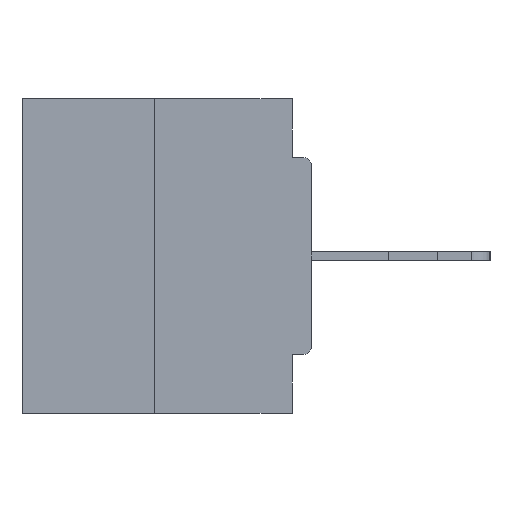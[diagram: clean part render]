
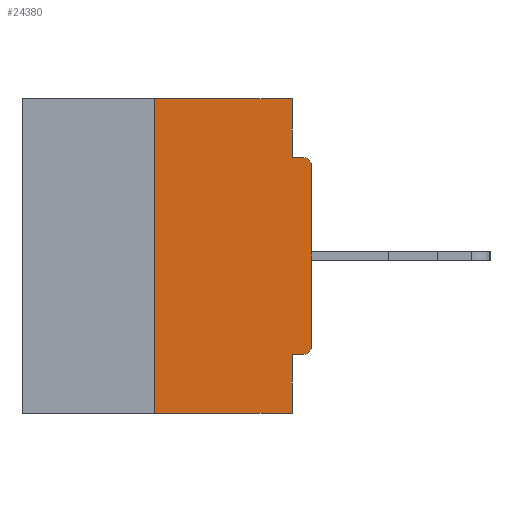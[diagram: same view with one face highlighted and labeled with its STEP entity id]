
A CAD part, left-side view. The second image highlights one B-rep face of the part: STEP entity #24380.
In plain terms, the highlighted planar face has unit normal (-1, 0, 0).
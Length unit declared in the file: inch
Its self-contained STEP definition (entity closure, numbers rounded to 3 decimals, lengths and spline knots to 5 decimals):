
#526 = ORIENTED_EDGE ( 'NONE', *, *, #13476, .T. ) ;
#1643 = DIRECTION ( 'NONE',  ( 0., 0., -1. ) ) ;
#1683 = CARTESIAN_POINT ( 'NONE',  ( 0., 0.46, 0. ) ) ;
#2128 = CARTESIAN_POINT ( 'NONE',  ( 0., 0.015, -0.4065 ) ) ;
#3144 = DIRECTION ( 'NONE',  ( 0., 1., 0. ) ) ;
#4366 = EDGE_CURVE ( 'NONE', #31973, #18933, #22867, .T. ) ;
#4422 = VERTEX_POINT ( 'NONE', #16410 ) ;
#5342 = VECTOR ( 'NONE', #16823, 39.37008 ) ;
#6203 = CARTESIAN_POINT ( 'NONE',  ( 0., 0.46, -0.5 ) ) ;
#6242 = ORIENTED_EDGE ( 'NONE', *, *, #23953, .F. ) ;
#6305 = PLANE ( 'NONE',  #9813 ) ;
#6490 = DIRECTION ( 'NONE',  ( 0., 0., -1. ) ) ;
#6770 = EDGE_LOOP ( 'NONE', ( #6242, #31537, #29741, #21243, #16342, #526, #17858, #17144, #28918, #13079 ) ) ;
#6972 = VECTOR ( 'NONE', #21790, 39.37008 ) ;
#6973 = LINE ( 'NONE', #30131, #22857 ) ;
#7571 = CARTESIAN_POINT ( 'NONE',  ( 0., 0., -0.1085 ) ) ;
#7632 = LINE ( 'NONE', #1683, #5342 ) ;
#8590 = VERTEX_POINT ( 'NONE', #9609 ) ;
#8731 = CARTESIAN_POINT ( 'NONE',  ( 0., 0.031, -0.4065 ) ) ;
#8762 = CARTESIAN_POINT ( 'NONE',  ( 0., 0.46, 0. ) ) ;
#8994 = CARTESIAN_POINT ( 'NONE',  ( 0., 0.015, -0.1085 ) ) ;
#9557 = EDGE_CURVE ( 'NONE', #23569, #20848, #27649, .T. ) ;
#9609 = CARTESIAN_POINT ( 'NONE',  ( 0., 0.031, -0.5 ) ) ;
#9813 = AXIS2_PLACEMENT_3D ( 'NONE', #8762, #31168, #1643 ) ;
#10285 = VERTEX_POINT ( 'NONE', #24629 ) ;
#10954 = CARTESIAN_POINT ( 'NONE',  ( 0., 0.25, 0. ) ) ;
#11067 = LINE ( 'NONE', #27284, #30048 ) ;
#12537 = CARTESIAN_POINT ( 'NONE',  ( 0., 0.031, -0.0935 ) ) ;
#13079 = ORIENTED_EDGE ( 'NONE', *, *, #22885, .F. ) ;
#13197 = VECTOR ( 'NONE', #15834, 39.37008 ) ;
#13476 = EDGE_CURVE ( 'NONE', #31973, #10285, #26076, .T. ) ;
#13555 = LINE ( 'NONE', #17165, #6972 ) ;
#13571 = VECTOR ( 'NONE', #3144, 39.37008 ) ;
#13758 = DIRECTION ( 'NONE',  ( 0., 0., 1. ) ) ;
#13796 = FACE_OUTER_BOUND ( 'NONE', #6770, .T. ) ;
#14166 = CARTESIAN_POINT ( 'NONE',  ( 0., 0.015, -0.3915 ) ) ;
#14942 = EDGE_CURVE ( 'NONE', #22138, #22860, #22891, .T. ) ;
#15296 = AXIS2_PLACEMENT_3D ( 'NONE', #8994, #31083, #6490 ) ;
#15401 = DIRECTION ( 'NONE',  ( 0., 0., -1. ) ) ;
#15822 = VERTEX_POINT ( 'NONE', #7571 ) ;
#15834 = DIRECTION ( 'NONE',  ( 0., -1., 0. ) ) ;
#16342 = ORIENTED_EDGE ( 'NONE', *, *, #4366, .F. ) ;
#16410 = CARTESIAN_POINT ( 'NONE',  ( 0., 0.031, 0. ) ) ;
#16823 = DIRECTION ( 'NONE',  ( 0., -1., 0. ) ) ;
#16846 = CIRCLE ( 'NONE', #15296, 0.015 ) ;
#17144 = ORIENTED_EDGE ( 'NONE', *, *, #28831, .T. ) ;
#17165 = CARTESIAN_POINT ( 'NONE',  ( 0., 0.031, -0.5 ) ) ;
#17858 = ORIENTED_EDGE ( 'NONE', *, *, #22026, .T. ) ;
#18138 = VECTOR ( 'NONE', #21350, 39.37008 ) ;
#18157 = EDGE_CURVE ( 'NONE', #18933, #8590, #13555, .T. ) ;
#18933 = VERTEX_POINT ( 'NONE', #8731 ) ;
#19499 = DIRECTION ( 'NONE',  ( 0., 0., 1. ) ) ;
#20848 = VERTEX_POINT ( 'NONE', #22329 ) ;
#21243 = ORIENTED_EDGE ( 'NONE', *, *, #18157, .F. ) ;
#21350 = DIRECTION ( 'NONE',  ( 0., -1., 0. ) ) ;
#21579 = AXIS2_PLACEMENT_3D ( 'NONE', #14166, #31510, #29457 ) ;
#21790 = DIRECTION ( 'NONE',  ( 0., 0., -1. ) ) ;
#22026 = EDGE_CURVE ( 'NONE', #10285, #15822, #11067, .T. ) ;
#22138 = VERTEX_POINT ( 'NONE', #12537 ) ;
#22329 = CARTESIAN_POINT ( 'NONE',  ( 0., 0.25, 0. ) ) ;
#22857 = VECTOR ( 'NONE', #15401, 39.37008 ) ;
#22860 = VERTEX_POINT ( 'NONE', #22880 ) ;
#22867 = LINE ( 'NONE', #30288, #13571 ) ;
#22880 = CARTESIAN_POINT ( 'NONE',  ( 0., 0.015, -0.0935 ) ) ;
#22885 = EDGE_CURVE ( 'NONE', #4422, #22138, #6973, .T. ) ;
#22891 = LINE ( 'NONE', #30683, #13197 ) ;
#23569 = VERTEX_POINT ( 'NONE', #24794 ) ;
#23771 = EDGE_CURVE ( 'NONE', #23569, #8590, #28168, .T. ) ;
#23953 = EDGE_CURVE ( 'NONE', #20848, #4422, #7632, .T. ) ;
#24380 = ADVANCED_FACE ( 'NONE', ( #13796 ), #6305, .F. ) ;
#24629 = CARTESIAN_POINT ( 'NONE',  ( 0., 0., -0.3915 ) ) ;
#24794 = CARTESIAN_POINT ( 'NONE',  ( 0., 0.25, -0.5 ) ) ;
#26076 = CIRCLE ( 'NONE', #21579, 0.015 ) ;
#27284 = CARTESIAN_POINT ( 'NONE',  ( 0., 0., 0. ) ) ;
#27649 = LINE ( 'NONE', #10954, #31910 ) ;
#28168 = LINE ( 'NONE', #6203, #18138 ) ;
#28831 = EDGE_CURVE ( 'NONE', #15822, #22860, #16846, .T. ) ;
#28918 = ORIENTED_EDGE ( 'NONE', *, *, #14942, .F. ) ;
#29457 = DIRECTION ( 'NONE',  ( 0., 0., -1. ) ) ;
#29741 = ORIENTED_EDGE ( 'NONE', *, *, #23771, .T. ) ;
#30048 = VECTOR ( 'NONE', #19499, 39.37008 ) ;
#30131 = CARTESIAN_POINT ( 'NONE',  ( 0., 0.031, 0. ) ) ;
#30288 = CARTESIAN_POINT ( 'NONE',  ( 0., 0., -0.4065 ) ) ;
#30683 = CARTESIAN_POINT ( 'NONE',  ( 0., 0., -0.0935 ) ) ;
#31083 = DIRECTION ( 'NONE',  ( -1., 0., 0. ) ) ;
#31168 = DIRECTION ( 'NONE',  ( 1., 0., 0. ) ) ;
#31510 = DIRECTION ( 'NONE',  ( -1., 0., 0. ) ) ;
#31537 = ORIENTED_EDGE ( 'NONE', *, *, #9557, .F. ) ;
#31910 = VECTOR ( 'NONE', #13758, 39.37008 ) ;
#31973 = VERTEX_POINT ( 'NONE', #2128 ) ;
